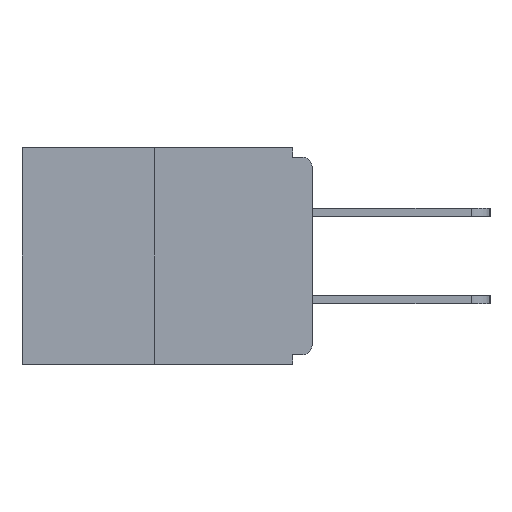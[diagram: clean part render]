
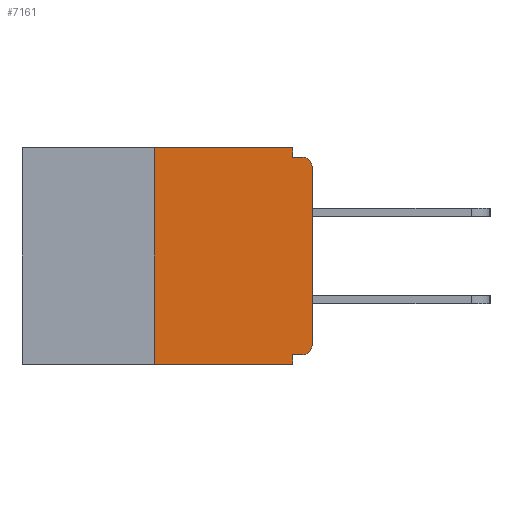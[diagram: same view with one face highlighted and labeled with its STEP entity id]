
A CAD part, left-side view. The second image highlights one B-rep face of the part: STEP entity #7161.
In plain terms, the highlighted planar face has unit normal (-1, 0, 0).
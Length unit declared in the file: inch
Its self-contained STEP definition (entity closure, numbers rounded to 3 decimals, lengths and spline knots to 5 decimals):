
#276 = ORIENTED_EDGE ( 'NONE', *, *, #3917, .F. ) ;
#325 = EDGE_CURVE ( 'NONE', #9626, #7927, #8031, .T. ) ;
#445 = CARTESIAN_POINT ( 'NONE',  ( 0., 0.015, -0.313 ) ) ;
#601 = CARTESIAN_POINT ( 'NONE',  ( 0., 0., -0.03 ) ) ;
#674 = EDGE_CURVE ( 'NONE', #13433, #2410, #12231, .T. ) ;
#858 = VECTOR ( 'NONE', #11947, 39.37008 ) ;
#913 = ORIENTED_EDGE ( 'NONE', *, *, #13155, .F. ) ;
#1167 = VERTEX_POINT ( 'NONE', #6365 ) ;
#1567 = DIRECTION ( 'NONE',  ( -1., 0., 0. ) ) ;
#1864 = DIRECTION ( 'NONE',  ( 0., 0., -1. ) ) ;
#2168 = ORIENTED_EDGE ( 'NONE', *, *, #8011, .F. ) ;
#2410 = VERTEX_POINT ( 'NONE', #601 ) ;
#2434 = ORIENTED_EDGE ( 'NONE', *, *, #8242, .T. ) ;
#2492 = EDGE_CURVE ( 'NONE', #2410, #12838, #18007, .T. ) ;
#2587 = CARTESIAN_POINT ( 'NONE',  ( 0., 0., -0.015 ) ) ;
#2686 = CARTESIAN_POINT ( 'NONE',  ( 0., 0.015, -0.03 ) ) ;
#2717 = DIRECTION ( 'NONE',  ( 1., 0., 0. ) ) ;
#2797 = EDGE_CURVE ( 'NONE', #1167, #14154, #13375, .T. ) ;
#3306 = CARTESIAN_POINT ( 'NONE',  ( 0., 0.031, -0.343 ) ) ;
#3597 = VERTEX_POINT ( 'NONE', #4455 ) ;
#3866 = LINE ( 'NONE', #4994, #13964 ) ;
#3917 = EDGE_CURVE ( 'NONE', #15948, #11881, #3866, .T. ) ;
#4455 = CARTESIAN_POINT ( 'NONE',  ( 0., 0.25, 0. ) ) ;
#4994 = CARTESIAN_POINT ( 'NONE',  ( 0., 0., -0.328 ) ) ;
#5087 = DIRECTION ( 'NONE',  ( 0., 1., 0. ) ) ;
#5209 = DIRECTION ( 'NONE',  ( 0., 0., -1. ) ) ;
#5341 = DIRECTION ( 'NONE',  ( 0., 0., -1. ) ) ;
#5736 = DIRECTION ( 'NONE',  ( 0., -1., 0. ) ) ;
#6094 = LINE ( 'NONE', #11675, #858 ) ;
#6338 = CARTESIAN_POINT ( 'NONE',  ( 0., 0.46, 0. ) ) ;
#6365 = CARTESIAN_POINT ( 'NONE',  ( 0., 0.031, 0. ) ) ;
#6743 = CARTESIAN_POINT ( 'NONE',  ( 0., 0., 0. ) ) ;
#7161 = ADVANCED_FACE ( 'NONE', ( #12416 ), #9665, .F. ) ;
#7213 = VECTOR ( 'NONE', #15201, 39.37008 ) ;
#7326 = VECTOR ( 'NONE', #5736, 39.37008 ) ;
#7357 = CARTESIAN_POINT ( 'NONE',  ( 0., 0.015, -0.328 ) ) ;
#7927 = VERTEX_POINT ( 'NONE', #3306 ) ;
#8011 = EDGE_CURVE ( 'NONE', #3597, #1167, #14647, .T. ) ;
#8012 = DIRECTION ( 'NONE',  ( 0., 0., 1. ) ) ;
#8031 = LINE ( 'NONE', #9757, #7326 ) ;
#8128 = LINE ( 'NONE', #17735, #10119 ) ;
#8242 = EDGE_CURVE ( 'NONE', #15948, #13433, #14697, .T. ) ;
#8291 = DIRECTION ( 'NONE',  ( 0., 0., -1. ) ) ;
#8366 = ORIENTED_EDGE ( 'NONE', *, *, #674, .T. ) ;
#8504 = DIRECTION ( 'NONE',  ( 0., 0., -1. ) ) ;
#8868 = VECTOR ( 'NONE', #17313, 39.37008 ) ;
#9626 = VERTEX_POINT ( 'NONE', #14289 ) ;
#9665 = PLANE ( 'NONE',  #15254 ) ;
#9729 = VECTOR ( 'NONE', #8012, 39.37008 ) ;
#9757 = CARTESIAN_POINT ( 'NONE',  ( 0., 0.46, -0.343 ) ) ;
#10119 = VECTOR ( 'NONE', #5209, 39.37008 ) ;
#10536 = EDGE_CURVE ( 'NONE', #11881, #7927, #8128, .T. ) ;
#11301 = CARTESIAN_POINT ( 'NONE',  ( 0., 0.031, -0.328 ) ) ;
#11675 = CARTESIAN_POINT ( 'NONE',  ( 0., 0.25, 0. ) ) ;
#11881 = VERTEX_POINT ( 'NONE', #11301 ) ;
#11947 = DIRECTION ( 'NONE',  ( 0., 0., 1. ) ) ;
#12214 = DIRECTION ( 'NONE',  ( -1., 0., 0. ) ) ;
#12231 = LINE ( 'NONE', #6743, #9729 ) ;
#12416 = FACE_OUTER_BOUND ( 'NONE', #13510, .T. ) ;
#12633 = ORIENTED_EDGE ( 'NONE', *, *, #325, .T. ) ;
#12838 = VERTEX_POINT ( 'NONE', #16496 ) ;
#12873 = ORIENTED_EDGE ( 'NONE', *, *, #2492, .T. ) ;
#13155 = EDGE_CURVE ( 'NONE', #9626, #3597, #6094, .T. ) ;
#13345 = ORIENTED_EDGE ( 'NONE', *, *, #2797, .F. ) ;
#13375 = LINE ( 'NONE', #14369, #16954 ) ;
#13433 = VERTEX_POINT ( 'NONE', #14103 ) ;
#13510 = EDGE_LOOP ( 'NONE', ( #2168, #913, #12633, #17602, #276, #2434, #8366, #12873, #17138, #13345 ) ) ;
#13964 = VECTOR ( 'NONE', #5087, 39.37008 ) ;
#14103 = CARTESIAN_POINT ( 'NONE',  ( 0., 0., -0.313 ) ) ;
#14154 = VERTEX_POINT ( 'NONE', #16719 ) ;
#14289 = CARTESIAN_POINT ( 'NONE',  ( 0., 0.25, -0.343 ) ) ;
#14369 = CARTESIAN_POINT ( 'NONE',  ( 0., 0.031, 0. ) ) ;
#14647 = LINE ( 'NONE', #6338, #8868 ) ;
#14697 = CIRCLE ( 'NONE', #17039, 0.015 ) ;
#14800 = AXIS2_PLACEMENT_3D ( 'NONE', #2686, #12214, #5341 ) ;
#15110 = LINE ( 'NONE', #2587, #7213 ) ;
#15201 = DIRECTION ( 'NONE',  ( 0., -1., 0. ) ) ;
#15238 = CARTESIAN_POINT ( 'NONE',  ( 0., 0.46, 0. ) ) ;
#15254 = AXIS2_PLACEMENT_3D ( 'NONE', #15238, #2717, #8291 ) ;
#15365 = EDGE_CURVE ( 'NONE', #14154, #12838, #15110, .T. ) ;
#15948 = VERTEX_POINT ( 'NONE', #7357 ) ;
#16496 = CARTESIAN_POINT ( 'NONE',  ( 0., 0.015, -0.015 ) ) ;
#16719 = CARTESIAN_POINT ( 'NONE',  ( 0., 0.031, -0.015 ) ) ;
#16954 = VECTOR ( 'NONE', #1864, 39.37008 ) ;
#17039 = AXIS2_PLACEMENT_3D ( 'NONE', #445, #1567, #8504 ) ;
#17138 = ORIENTED_EDGE ( 'NONE', *, *, #15365, .F. ) ;
#17313 = DIRECTION ( 'NONE',  ( 0., -1., 0. ) ) ;
#17602 = ORIENTED_EDGE ( 'NONE', *, *, #10536, .F. ) ;
#17735 = CARTESIAN_POINT ( 'NONE',  ( 0., 0.031, -0.343 ) ) ;
#18007 = CIRCLE ( 'NONE', #14800, 0.015 ) ;
